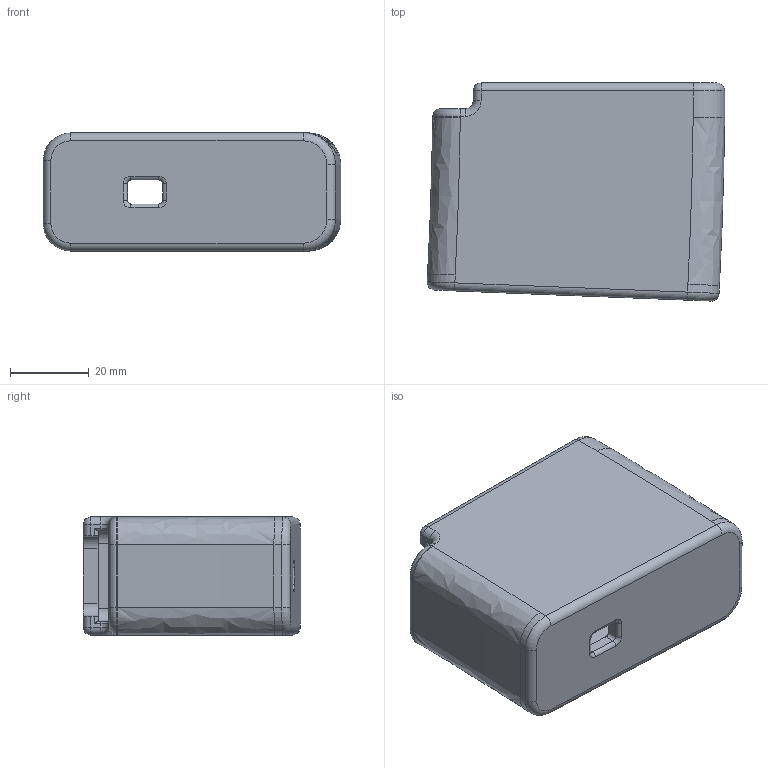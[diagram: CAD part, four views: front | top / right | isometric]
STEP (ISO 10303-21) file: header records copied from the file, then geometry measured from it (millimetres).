
FILE_DESCRIPTION(/* description */ (''),/* implementation_level */ '2;1');
FILE_NAME(/* name */ 'cff23bac-a708-457e-b166-bc910e2813bf.stp',/* time_stamp */ '2019-04-30T20:31:59-04:00',/* author */ ('suzuki450ltr'),/* organization */ (''),/* preprocessor_version */ 'ST-DEVELOPER v18',/* originating_system */ 'Autodesk Translation Framework v8.2.0.1029',/* authorisation */ '');
FILE_SCHEMA (('AUTOMOTIVE_DESIGN { 1 0 10303 214 3 1 1 }'));
Length unit declared in the file: millimetre
Products named in the file (1): Lancer 30RD Mag Extension
Bounding box: 75.36 x 55.23 x 29.9 mm (x, y, z)
Volume: 57805.9 mm3; surface area: 22549.6 mm2
Topology: 1 solids, 1 shells, 215 faces, 508 edges, 292 vertices
Faces by surface type: cylinder 93, bspline 42, plane 42, torus 28, cone 6, sphere 4
Full cylindrical faces by diameter (mm): 3 x1
Entity records: 6706 total; most frequent: CARTESIAN_POINT 1795, DIRECTION 1078, ORIENTED_EDGE 1008, EDGE_CURVE 504, AXIS2_PLACEMENT_3D 434, VERTEX_POINT 292, CIRCLE 252, EDGE_LOOP 218
